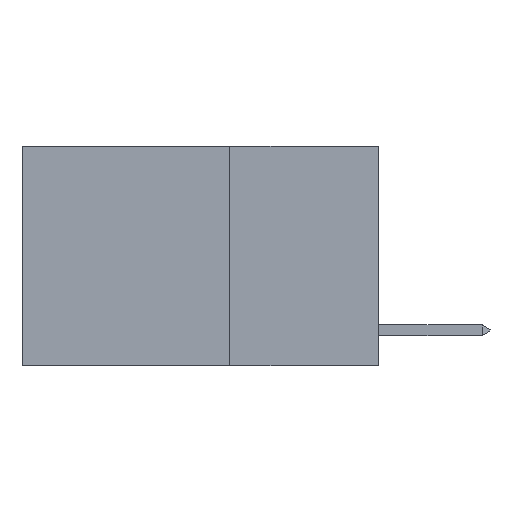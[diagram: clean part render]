
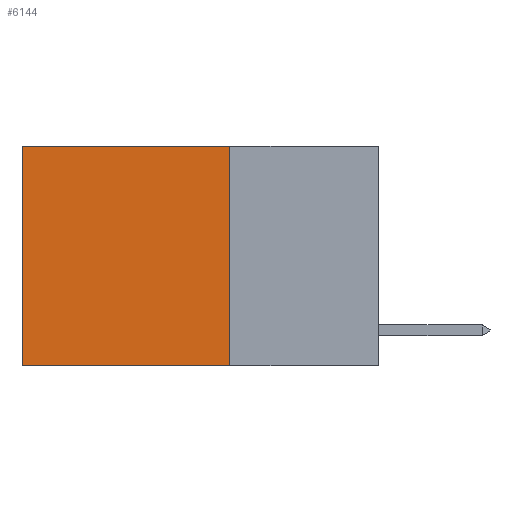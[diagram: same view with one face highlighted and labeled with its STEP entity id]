
A CAD part, left-side view. The second image highlights one B-rep face of the part: STEP entity #6144.
In plain terms, the highlighted planar face has unit normal (-1, 0, 0).
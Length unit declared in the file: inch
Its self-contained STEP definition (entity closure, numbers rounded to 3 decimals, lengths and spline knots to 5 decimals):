
#120 = FACE_OUTER_BOUND ( 'NONE', #14349, .T. ) ;
#188 = VECTOR ( 'NONE', #19369, 39.37008 ) ;
#313 = VECTOR ( 'NONE', #7403, 39.37008 ) ;
#811 = EDGE_CURVE ( 'NONE', #5199, #7086, #5380, .T. ) ;
#3746 = CARTESIAN_POINT ( 'NONE',  ( 0.2625, 0.25, 0. ) ) ;
#4124 = DIRECTION ( 'NONE',  ( 0., 0., -1. ) ) ;
#5199 = VERTEX_POINT ( 'NONE', #9289 ) ;
#5380 = LINE ( 'NONE', #3746, #313 ) ;
#5622 = EDGE_CURVE ( 'NONE', #7086, #15811, #10615, .T. ) ;
#5819 = DIRECTION ( 'NONE',  ( 0., 1., 0. ) ) ;
#5849 = DIRECTION ( 'NONE',  ( 0., 0., -1. ) ) ;
#6144 = ADVANCED_FACE ( 'NONE', ( #120 ), #10147, .F. ) ;
#6655 = VECTOR ( 'NONE', #5849, 39.37008 ) ;
#7086 = VERTEX_POINT ( 'NONE', #9560 ) ;
#7403 = DIRECTION ( 'NONE',  ( 0., 1., 0. ) ) ;
#7617 = CARTESIAN_POINT ( 'NONE',  ( 0.2625, 0.25, 0. ) ) ;
#8241 = AXIS2_PLACEMENT_3D ( 'NONE', #17556, #13161, #4124 ) ;
#9289 = CARTESIAN_POINT ( 'NONE',  ( 0.2625, 0.25, 0. ) ) ;
#9345 = LINE ( 'NONE', #16304, #16814 ) ;
#9560 = CARTESIAN_POINT ( 'NONE',  ( 0.2625, 0.6, 0. ) ) ;
#10078 = CARTESIAN_POINT ( 'NONE',  ( 0.2625, 0.25, -0.37 ) ) ;
#10147 = PLANE ( 'NONE',  #8241 ) ;
#10303 = CARTESIAN_POINT ( 'NONE',  ( 0.2625, 0.6, 0. ) ) ;
#10615 = LINE ( 'NONE', #10303, #6655 ) ;
#10925 = ORIENTED_EDGE ( 'NONE', *, *, #5622, .T. ) ;
#12418 = ORIENTED_EDGE ( 'NONE', *, *, #18875, .F. ) ;
#13161 = DIRECTION ( 'NONE',  ( 1., 0., 0. ) ) ;
#14140 = CARTESIAN_POINT ( 'NONE',  ( 0.2625, 0.6, -0.37 ) ) ;
#14349 = EDGE_LOOP ( 'NONE', ( #10925, #12418, #14475, #14589 ) ) ;
#14475 = ORIENTED_EDGE ( 'NONE', *, *, #16117, .F. ) ;
#14589 = ORIENTED_EDGE ( 'NONE', *, *, #811, .T. ) ;
#15296 = VERTEX_POINT ( 'NONE', #10078 ) ;
#15811 = VERTEX_POINT ( 'NONE', #14140 ) ;
#16117 = EDGE_CURVE ( 'NONE', #5199, #15296, #16742, .T. ) ;
#16304 = CARTESIAN_POINT ( 'NONE',  ( 0.2625, 0.25, -0.37 ) ) ;
#16742 = LINE ( 'NONE', #7617, #188 ) ;
#16814 = VECTOR ( 'NONE', #5819, 39.37008 ) ;
#17556 = CARTESIAN_POINT ( 'NONE',  ( 0.2625, 0.25, 0. ) ) ;
#18875 = EDGE_CURVE ( 'NONE', #15296, #15811, #9345, .T. ) ;
#19369 = DIRECTION ( 'NONE',  ( 0., 0., -1. ) ) ;
